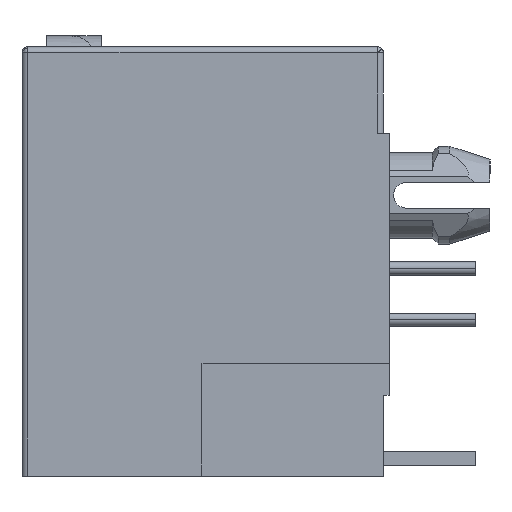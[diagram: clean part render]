
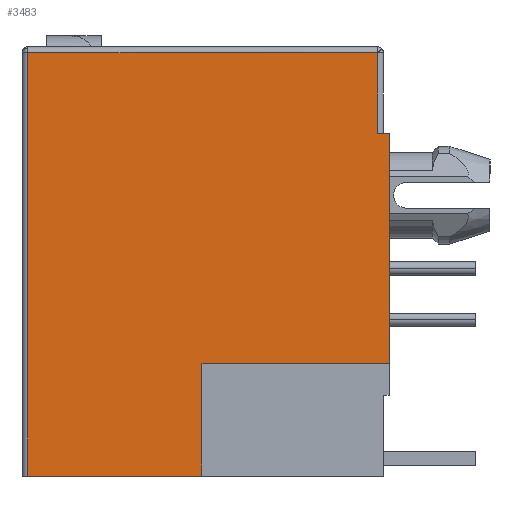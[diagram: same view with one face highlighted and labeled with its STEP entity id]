
A CAD part, left-side view. The second image highlights one B-rep face of the part: STEP entity #3483.
In plain terms, the highlighted planar face has unit normal (-1, 0, 0).
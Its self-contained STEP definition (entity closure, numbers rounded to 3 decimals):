
#79 = ORIENTED_EDGE ( 'NONE', *, *, #33568, .T. ) ;
#1824 = ORIENTED_EDGE ( 'NONE', *, *, #26675, .T. ) ;
#2955 = CARTESIAN_POINT ( 'NONE',  ( -8.025, 5.925, 7.325 ) ) ;
#3483 = ADVANCED_FACE ( 'NONE', ( #48109 ), #36476, .T. ) ;
#3814 = DIRECTION ( 'NONE',  ( 0., 0., 1. ) ) ;
#5093 = CARTESIAN_POINT ( 'NONE',  ( -8.025, 0., 7.325 ) ) ;
#5405 = LINE ( 'NONE', #55848, #20456 ) ;
#5736 = CARTESIAN_POINT ( 'NONE',  ( -8.025, 5.925, 26.949 ) ) ;
#6507 = CARTESIAN_POINT ( 'NONE',  ( -8.025, 5.925, -7.375 ) ) ;
#6661 = CARTESIAN_POINT ( 'NONE',  ( -8.025, -6.225, 4.525 ) ) ;
#7236 = ORIENTED_EDGE ( 'NONE', *, *, #48326, .T. ) ;
#7398 = LINE ( 'NONE', #12787, #48197 ) ;
#7639 = AXIS2_PLACEMENT_3D ( 'NONE', #9255, #19057, #53069 ) ;
#7753 = VECTOR ( 'NONE', #11216, 1000. ) ;
#9255 = CARTESIAN_POINT ( 'NONE',  ( -8.025, 0., 0. ) ) ;
#9436 = EDGE_CURVE ( 'NONE', #11521, #53523, #58367, .T. ) ;
#11125 = CARTESIAN_POINT ( 'NONE',  ( -8.025, -0.125, -3.475 ) ) ;
#11216 = DIRECTION ( 'NONE',  ( 0., 0., 1. ) ) ;
#11246 = VECTOR ( 'NONE', #41653, 1000. ) ;
#11335 = VERTEX_POINT ( 'NONE', #50595 ) ;
#11521 = VERTEX_POINT ( 'NONE', #41894 ) ;
#12787 = CARTESIAN_POINT ( 'NONE',  ( -8.025, 0., -7.375 ) ) ;
#13343 = LINE ( 'NONE', #5093, #18583 ) ;
#13925 = CARTESIAN_POINT ( 'NONE',  ( -8.025, -0.125, 0. ) ) ;
#16889 = VECTOR ( 'NONE', #30232, 1000. ) ;
#17212 = DIRECTION ( 'NONE',  ( 0., -1., 0. ) ) ;
#17912 = CARTESIAN_POINT ( 'NONE',  ( -8.025, -6.625, -3.475 ) ) ;
#18583 = VECTOR ( 'NONE', #39030, 1000. ) ;
#19057 = DIRECTION ( 'NONE',  ( -1., 0., 0. ) ) ;
#20456 = VECTOR ( 'NONE', #41841, 1000. ) ;
#20690 = CARTESIAN_POINT ( 'NONE',  ( -8.025, -6.225, 7.325 ) ) ;
#21436 = ORIENTED_EDGE ( 'NONE', *, *, #50461, .T. ) ;
#22963 = EDGE_CURVE ( 'NONE', #30405, #28827, #29638, .T. ) ;
#23556 = CARTESIAN_POINT ( 'NONE',  ( -8.025, -6.225, 0. ) ) ;
#25188 = LINE ( 'NONE', #36510, #50861 ) ;
#26675 = EDGE_CURVE ( 'NONE', #53523, #28797, #62648, .T. ) ;
#27546 = CARTESIAN_POINT ( 'NONE',  ( -8.025, 0., -3.475 ) ) ;
#27940 = ORIENTED_EDGE ( 'NONE', *, *, #22963, .F. ) ;
#28797 = VERTEX_POINT ( 'NONE', #17912 ) ;
#28827 = VERTEX_POINT ( 'NONE', #2955 ) ;
#29638 = LINE ( 'NONE', #5736, #7753 ) ;
#29850 = VERTEX_POINT ( 'NONE', #20690 ) ;
#30232 = DIRECTION ( 'NONE',  ( 0., 0., 1. ) ) ;
#30405 = VERTEX_POINT ( 'NONE', #6507 ) ;
#33568 = EDGE_CURVE ( 'NONE', #61645, #29850, #35761, .T. ) ;
#35761 = LINE ( 'NONE', #23556, #16889 ) ;
#36476 = PLANE ( 'NONE',  #7639 ) ;
#36510 = CARTESIAN_POINT ( 'NONE',  ( -8.025, -6.625, 0. ) ) ;
#37114 = ORIENTED_EDGE ( 'NONE', *, *, #61719, .T. ) ;
#39030 = DIRECTION ( 'NONE',  ( 0., 1., 0. ) ) ;
#41653 = DIRECTION ( 'NONE',  ( 0., -1., 0. ) ) ;
#41841 = DIRECTION ( 'NONE',  ( 0., 1., 0. ) ) ;
#41861 = ORIENTED_EDGE ( 'NONE', *, *, #57373, .T. ) ;
#41894 = CARTESIAN_POINT ( 'NONE',  ( -8.025, -0.125, -7.375 ) ) ;
#42989 = EDGE_LOOP ( 'NONE', ( #51779, #1824, #41861, #37114, #79, #7236, #27940, #21436 ) ) ;
#46203 = VECTOR ( 'NONE', #3814, 1000. ) ;
#46623 = DIRECTION ( 'NONE',  ( 0., 0., 1. ) ) ;
#48109 = FACE_OUTER_BOUND ( 'NONE', #42989, .T. ) ;
#48197 = VECTOR ( 'NONE', #17212, 1000. ) ;
#48326 = EDGE_CURVE ( 'NONE', #29850, #28827, #13343, .T. ) ;
#50461 = EDGE_CURVE ( 'NONE', #30405, #11521, #7398, .T. ) ;
#50595 = CARTESIAN_POINT ( 'NONE',  ( -8.025, -6.625, 4.525 ) ) ;
#50861 = VECTOR ( 'NONE', #46623, 1000. ) ;
#51779 = ORIENTED_EDGE ( 'NONE', *, *, #9436, .T. ) ;
#53069 = DIRECTION ( 'NONE',  ( 0., -1., 0. ) ) ;
#53523 = VERTEX_POINT ( 'NONE', #11125 ) ;
#55848 = CARTESIAN_POINT ( 'NONE',  ( -8.025, -6.635, 4.525 ) ) ;
#57373 = EDGE_CURVE ( 'NONE', #28797, #11335, #25188, .T. ) ;
#58367 = LINE ( 'NONE', #13925, #46203 ) ;
#61645 = VERTEX_POINT ( 'NONE', #6661 ) ;
#61719 = EDGE_CURVE ( 'NONE', #11335, #61645, #5405, .T. ) ;
#62648 = LINE ( 'NONE', #27546, #11246 ) ;
